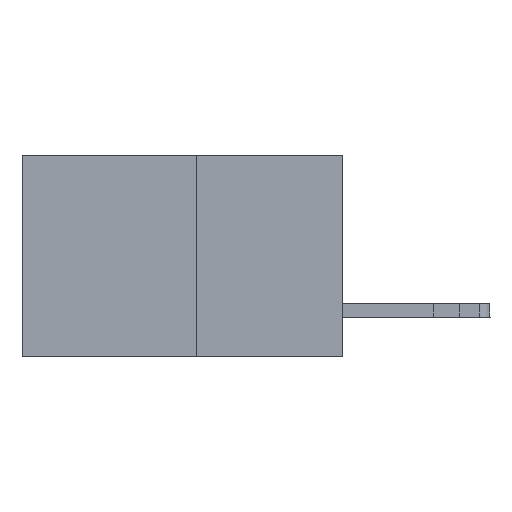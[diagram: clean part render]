
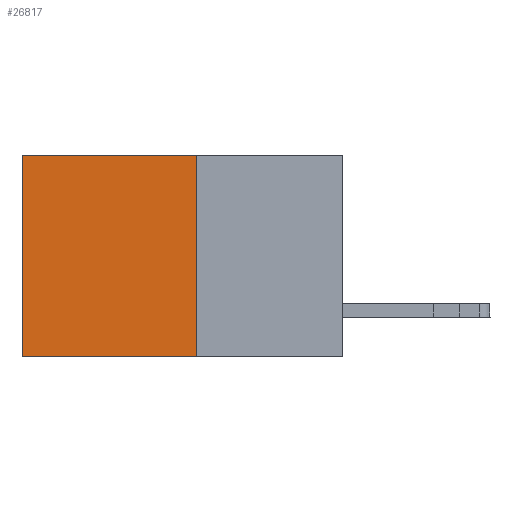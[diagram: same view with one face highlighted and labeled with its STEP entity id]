
A CAD part, left-side view. The second image highlights one B-rep face of the part: STEP entity #26817.
In plain terms, the highlighted planar face has unit normal (-1, 0, 0).
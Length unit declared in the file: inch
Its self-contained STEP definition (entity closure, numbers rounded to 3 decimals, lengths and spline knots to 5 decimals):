
#2510 = DIRECTION ( 'NONE',  ( 0., 1., 0. ) ) ;
#3564 = ORIENTED_EDGE ( 'NONE', *, *, #8770, .T. ) ;
#5069 = VECTOR ( 'NONE', #28153, 39.37008 ) ;
#5915 = DIRECTION ( 'NONE',  ( 0., 0., -1. ) ) ;
#6243 = ORIENTED_EDGE ( 'NONE', *, *, #24179, .F. ) ;
#7391 = VERTEX_POINT ( 'NONE', #16254 ) ;
#7835 = CARTESIAN_POINT ( 'NONE',  ( 0.277, 0.27, 0. ) ) ;
#8770 = EDGE_CURVE ( 'NONE', #19241, #7391, #19052, .T. ) ;
#10020 = FACE_OUTER_BOUND ( 'NONE', #16193, .T. ) ;
#10074 = CARTESIAN_POINT ( 'NONE',  ( 0.277, 0.59, -0.37 ) ) ;
#10808 = CARTESIAN_POINT ( 'NONE',  ( 0.277, 0.27, -0.37 ) ) ;
#12451 = PLANE ( 'NONE',  #23840 ) ;
#12979 = ORIENTED_EDGE ( 'NONE', *, *, #20621, .F. ) ;
#13648 = EDGE_CURVE ( 'NONE', #7391, #27614, #22039, .T. ) ;
#14570 = CARTESIAN_POINT ( 'NONE',  ( 0.277, 0.27, 0. ) ) ;
#14767 = LINE ( 'NONE', #10808, #16278 ) ;
#16193 = EDGE_LOOP ( 'NONE', ( #22628, #6243, #12979, #3564 ) ) ;
#16254 = CARTESIAN_POINT ( 'NONE',  ( 0.277, 0.59, 0. ) ) ;
#16278 = VECTOR ( 'NONE', #26904, 39.37008 ) ;
#16742 = CARTESIAN_POINT ( 'NONE',  ( 0.277, 0.59, -0.37 ) ) ;
#19033 = CARTESIAN_POINT ( 'NONE',  ( 0.277, 0.27, -0.37 ) ) ;
#19052 = LINE ( 'NONE', #7835, #5069 ) ;
#19241 = VERTEX_POINT ( 'NONE', #14570 ) ;
#20621 = EDGE_CURVE ( 'NONE', #19241, #21831, #14767, .T. ) ;
#21814 = VECTOR ( 'NONE', #2510, 39.37008 ) ;
#21831 = VERTEX_POINT ( 'NONE', #25065 ) ;
#22039 = LINE ( 'NONE', #10074, #27183 ) ;
#22628 = ORIENTED_EDGE ( 'NONE', *, *, #13648, .T. ) ;
#23840 = AXIS2_PLACEMENT_3D ( 'NONE', #24566, #26696, #5915 ) ;
#24179 = EDGE_CURVE ( 'NONE', #21831, #27614, #27847, .T. ) ;
#24566 = CARTESIAN_POINT ( 'NONE',  ( 0.277, 0.27, -0.37 ) ) ;
#25065 = CARTESIAN_POINT ( 'NONE',  ( 0.277, 0.27, -0.37 ) ) ;
#26696 = DIRECTION ( 'NONE',  ( 1., 0., 0. ) ) ;
#26817 = ADVANCED_FACE ( 'NONE', ( #10020 ), #12451, .F. ) ;
#26904 = DIRECTION ( 'NONE',  ( 0., 0., -1. ) ) ;
#27183 = VECTOR ( 'NONE', #28894, 39.37008 ) ;
#27614 = VERTEX_POINT ( 'NONE', #16742 ) ;
#27847 = LINE ( 'NONE', #19033, #21814 ) ;
#28153 = DIRECTION ( 'NONE',  ( 0., 1., 0. ) ) ;
#28894 = DIRECTION ( 'NONE',  ( 0., 0., -1. ) ) ;
